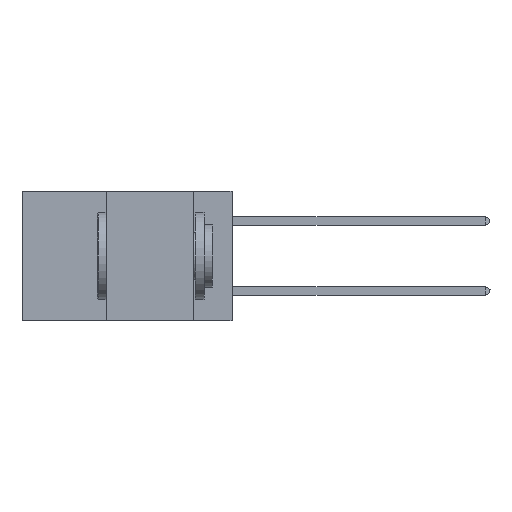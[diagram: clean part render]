
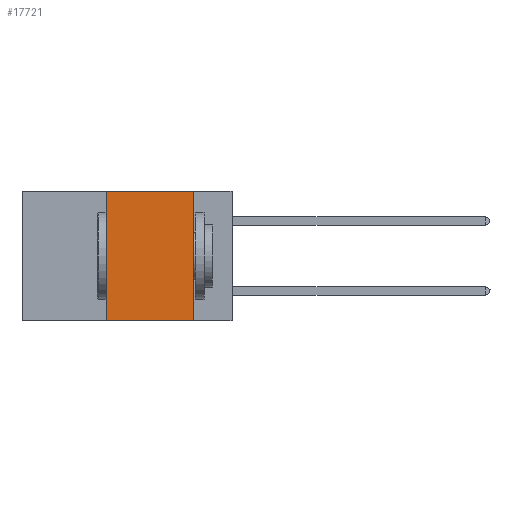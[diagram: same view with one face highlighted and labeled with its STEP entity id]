
A CAD part, left-side view. The second image highlights one B-rep face of the part: STEP entity #17721.
In plain terms, the highlighted planar face has unit normal (-1, 0, 0).
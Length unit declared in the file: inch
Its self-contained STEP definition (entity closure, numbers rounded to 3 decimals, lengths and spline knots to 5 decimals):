
#938 = CARTESIAN_POINT ( 'NONE',  ( 0., 0.6, 0. ) ) ;
#1017 = DIRECTION ( 'NONE',  ( 1., 0., 0. ) ) ;
#1166 = LINE ( 'NONE', #6187, #5505 ) ;
#1717 = EDGE_CURVE ( 'NONE', #8899, #3088, #3994, .T. ) ;
#2072 = ORIENTED_EDGE ( 'NONE', *, *, #17610, .F. ) ;
#2168 = VECTOR ( 'NONE', #22271, 39.37008 ) ;
#3088 = VERTEX_POINT ( 'NONE', #21183 ) ;
#3567 = EDGE_CURVE ( 'NONE', #7891, #5806, #11150, .T. ) ;
#3994 = LINE ( 'NONE', #13862, #13589 ) ;
#4943 = FACE_OUTER_BOUND ( 'NONE', #23073, .T. ) ;
#5300 = CARTESIAN_POINT ( 'NONE',  ( 0., 0.36, 0. ) ) ;
#5505 = VECTOR ( 'NONE', #19202, 39.37008 ) ;
#5806 = VERTEX_POINT ( 'NONE', #9379 ) ;
#6089 = VECTOR ( 'NONE', #14204, 39.37008 ) ;
#6187 = CARTESIAN_POINT ( 'NONE',  ( 0., 0.6, 0. ) ) ;
#6211 = AXIS2_PLACEMENT_3D ( 'NONE', #938, #1017, #15886 ) ;
#6430 = CARTESIAN_POINT ( 'NONE',  ( 0., 0.36, -0.37 ) ) ;
#6433 = PLANE ( 'NONE',  #6211 ) ;
#7891 = VERTEX_POINT ( 'NONE', #6430 ) ;
#8899 = VERTEX_POINT ( 'NONE', #16942 ) ;
#9379 = CARTESIAN_POINT ( 'NONE',  ( 0., 0.36, 0. ) ) ;
#10934 = EDGE_CURVE ( 'NONE', #7891, #3088, #17746, .T. ) ;
#11150 = LINE ( 'NONE', #5300, #2168 ) ;
#12974 = ORIENTED_EDGE ( 'NONE', *, *, #10934, .T. ) ;
#13589 = VECTOR ( 'NONE', #15716, 39.37008 ) ;
#13862 = CARTESIAN_POINT ( 'NONE',  ( 0., 0.11, 0. ) ) ;
#14204 = DIRECTION ( 'NONE',  ( 0., -1., 0. ) ) ;
#15716 = DIRECTION ( 'NONE',  ( 0., 0., -1. ) ) ;
#15886 = DIRECTION ( 'NONE',  ( 0., 0., -1. ) ) ;
#15985 = CARTESIAN_POINT ( 'NONE',  ( 0., 0.6, -0.37 ) ) ;
#16942 = CARTESIAN_POINT ( 'NONE',  ( 0., 0.11, 0. ) ) ;
#16985 = ORIENTED_EDGE ( 'NONE', *, *, #1717, .F. ) ;
#17610 = EDGE_CURVE ( 'NONE', #5806, #8899, #1166, .T. ) ;
#17721 = ADVANCED_FACE ( 'NONE', ( #4943 ), #6433, .F. ) ;
#17746 = LINE ( 'NONE', #15985, #6089 ) ;
#18243 = ORIENTED_EDGE ( 'NONE', *, *, #3567, .F. ) ;
#19202 = DIRECTION ( 'NONE',  ( 0., -1., 0. ) ) ;
#21183 = CARTESIAN_POINT ( 'NONE',  ( 0., 0.11, -0.37 ) ) ;
#22271 = DIRECTION ( 'NONE',  ( 0., 0., 1. ) ) ;
#23073 = EDGE_LOOP ( 'NONE', ( #16985, #2072, #18243, #12974 ) ) ;
